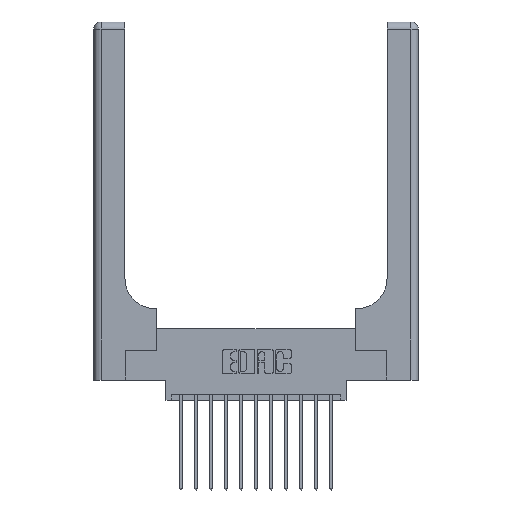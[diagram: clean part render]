
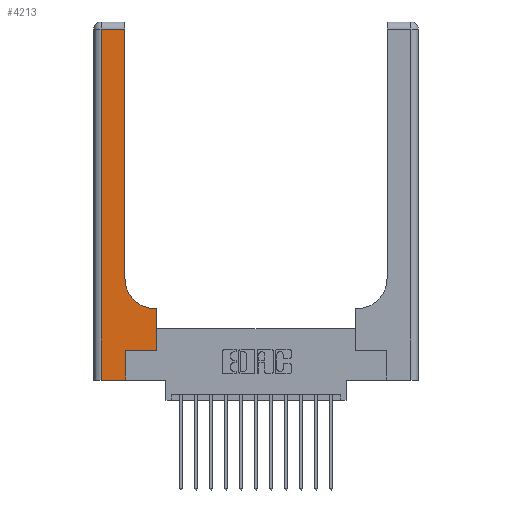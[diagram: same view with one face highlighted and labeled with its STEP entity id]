
A CAD part, top view. The second image highlights one B-rep face of the part: STEP entity #4213.
In plain terms, the highlighted planar face has unit normal (0, 0, 1).
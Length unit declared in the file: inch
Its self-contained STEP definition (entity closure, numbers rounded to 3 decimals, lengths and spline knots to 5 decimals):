
#108 = LINE ( 'NONE', #3521, #7001 ) ;
#132 = VECTOR ( 'NONE', #3655, 39.37008 ) ;
#466 = DIRECTION ( 'NONE',  ( 0., 0., -1. ) ) ;
#785 = CARTESIAN_POINT ( 'NONE',  ( 0.528, 0.6, 0.37 ) ) ;
#1091 = ORIENTED_EDGE ( 'NONE', *, *, #14571, .T. ) ;
#1348 = ORIENTED_EDGE ( 'NONE', *, *, #4970, .T. ) ;
#1455 = VERTEX_POINT ( 'NONE', #3039 ) ;
#1484 = LINE ( 'NONE', #12244, #14382 ) ;
#1774 = DIRECTION ( 'NONE',  ( 0., 1., 0. ) ) ;
#1775 = EDGE_CURVE ( 'NONE', #5137, #8165, #16695, .T. ) ;
#1912 = VERTEX_POINT ( 'NONE', #14393 ) ;
#1943 = VERTEX_POINT ( 'NONE', #10589 ) ;
#2140 = VERTEX_POINT ( 'NONE', #5893 ) ;
#2846 = DIRECTION ( 'NONE',  ( 0., 1., 0. ) ) ;
#2883 = VERTEX_POINT ( 'NONE', #15592 ) ;
#3039 = CARTESIAN_POINT ( 'NONE',  ( 0.06, 2.94, 0.37 ) ) ;
#3317 = VERTEX_POINT ( 'NONE', #15241 ) ;
#3411 = VECTOR ( 'NONE', #2846, 39.37008 ) ;
#3521 = CARTESIAN_POINT ( 'NONE',  ( 0., 0., 0.37 ) ) ;
#3573 = CIRCLE ( 'NONE', #16292, 0.25 ) ;
#3598 = LINE ( 'NONE', #8787, #132 ) ;
#3655 = DIRECTION ( 'NONE',  ( -1., 0., 0. ) ) ;
#3744 = LINE ( 'NONE', #15374, #10203 ) ;
#4106 = AXIS2_PLACEMENT_3D ( 'NONE', #5614, #466, #9510 ) ;
#4213 = ADVANCED_FACE ( 'NONE', ( #6364 ), #8212, .F. ) ;
#4263 = CARTESIAN_POINT ( 'NONE',  ( 0.26, 3., 0.37 ) ) ;
#4506 = CARTESIAN_POINT ( 'NONE',  ( 0.51, 0.6, 0.37 ) ) ;
#4811 = DIRECTION ( 'NONE',  ( 1., 0., 0. ) ) ;
#4970 = EDGE_CURVE ( 'NONE', #1455, #2140, #1484, .T. ) ;
#5137 = VERTEX_POINT ( 'NONE', #785 ) ;
#5180 = DIRECTION ( 'NONE',  ( -1., 0., 0. ) ) ;
#5333 = DIRECTION ( 'NONE',  ( 0., 0., -1. ) ) ;
#5614 = CARTESIAN_POINT ( 'NONE',  ( 0., 3., 0.37 ) ) ;
#5846 = VECTOR ( 'NONE', #1774, 39.37008 ) ;
#5893 = CARTESIAN_POINT ( 'NONE',  ( 0.06, 0., 0.37 ) ) ;
#6278 = EDGE_CURVE ( 'NONE', #8165, #1912, #3573, .T. ) ;
#6364 = FACE_OUTER_BOUND ( 'NONE', #12385, .T. ) ;
#7001 = VECTOR ( 'NONE', #4811, 39.37008 ) ;
#7003 = ORIENTED_EDGE ( 'NONE', *, *, #1775, .T. ) ;
#7437 = ORIENTED_EDGE ( 'NONE', *, *, #6278, .T. ) ;
#7697 = DIRECTION ( 'NONE',  ( 1., 0., 0. ) ) ;
#8165 = VERTEX_POINT ( 'NONE', #4506 ) ;
#8212 = PLANE ( 'NONE',  #4106 ) ;
#8480 = LINE ( 'NONE', #4263, #5846 ) ;
#8787 = CARTESIAN_POINT ( 'NONE',  ( 0., 2.94, 0.37 ) ) ;
#9372 = VERTEX_POINT ( 'NONE', #10676 ) ;
#9510 = DIRECTION ( 'NONE',  ( -1., 0., 0. ) ) ;
#9897 = VECTOR ( 'NONE', #5180, 39.37008 ) ;
#9909 = CARTESIAN_POINT ( 'NONE',  ( 0.265, 0., 0.37 ) ) ;
#10203 = VECTOR ( 'NONE', #7697, 39.37008 ) ;
#10443 = VECTOR ( 'NONE', #11197, 39.37008 ) ;
#10540 = EDGE_CURVE ( 'NONE', #1912, #9372, #8480, .T. ) ;
#10575 = CARTESIAN_POINT ( 'NONE',  ( 0.528, 0.25, 0.37 ) ) ;
#10589 = CARTESIAN_POINT ( 'NONE',  ( 0.528, 0.25, 0.37 ) ) ;
#10676 = CARTESIAN_POINT ( 'NONE',  ( 0.26, 2.94, 0.37 ) ) ;
#11138 = EDGE_CURVE ( 'NONE', #1943, #5137, #13282, .T. ) ;
#11197 = DIRECTION ( 'NONE',  ( 0., 1., 0. ) ) ;
#11270 = ORIENTED_EDGE ( 'NONE', *, *, #11138, .T. ) ;
#12244 = CARTESIAN_POINT ( 'NONE',  ( 0.06, 3., 0.37 ) ) ;
#12385 = EDGE_LOOP ( 'NONE', ( #14023, #15527, #1348, #13646, #1091, #13556, #11270, #7003, #7437 ) ) ;
#12612 = EDGE_CURVE ( 'NONE', #9372, #1455, #3598, .T. ) ;
#12887 = CARTESIAN_POINT ( 'NONE',  ( 0.26, 0.6, 0.37 ) ) ;
#13038 = CARTESIAN_POINT ( 'NONE',  ( 0.51, 0.85, 0.37 ) ) ;
#13282 = LINE ( 'NONE', #10575, #3411 ) ;
#13538 = DIRECTION ( 'NONE',  ( 0., -1., 0. ) ) ;
#13556 = ORIENTED_EDGE ( 'NONE', *, *, #15841, .T. ) ;
#13646 = ORIENTED_EDGE ( 'NONE', *, *, #14598, .T. ) ;
#13835 = LINE ( 'NONE', #9909, #10443 ) ;
#14023 = ORIENTED_EDGE ( 'NONE', *, *, #10540, .T. ) ;
#14326 = DIRECTION ( 'NONE',  ( 1., 0., 0. ) ) ;
#14382 = VECTOR ( 'NONE', #13538, 39.37008 ) ;
#14393 = CARTESIAN_POINT ( 'NONE',  ( 0.26, 0.85, 0.37 ) ) ;
#14571 = EDGE_CURVE ( 'NONE', #3317, #2883, #13835, .T. ) ;
#14598 = EDGE_CURVE ( 'NONE', #2140, #3317, #108, .T. ) ;
#15241 = CARTESIAN_POINT ( 'NONE',  ( 0.265, 0., 0.37 ) ) ;
#15374 = CARTESIAN_POINT ( 'NONE',  ( 0.265, 0.25, 0.37 ) ) ;
#15527 = ORIENTED_EDGE ( 'NONE', *, *, #12612, .T. ) ;
#15592 = CARTESIAN_POINT ( 'NONE',  ( 0.265, 0.25, 0.37 ) ) ;
#15841 = EDGE_CURVE ( 'NONE', #2883, #1943, #3744, .T. ) ;
#16292 = AXIS2_PLACEMENT_3D ( 'NONE', #13038, #5333, #14326 ) ;
#16695 = LINE ( 'NONE', #12887, #9897 ) ;
